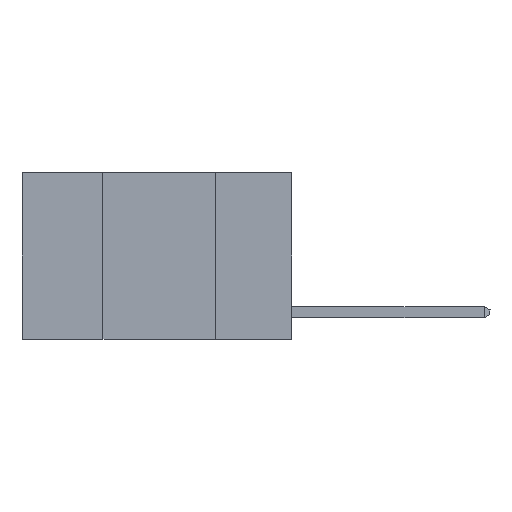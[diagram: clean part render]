
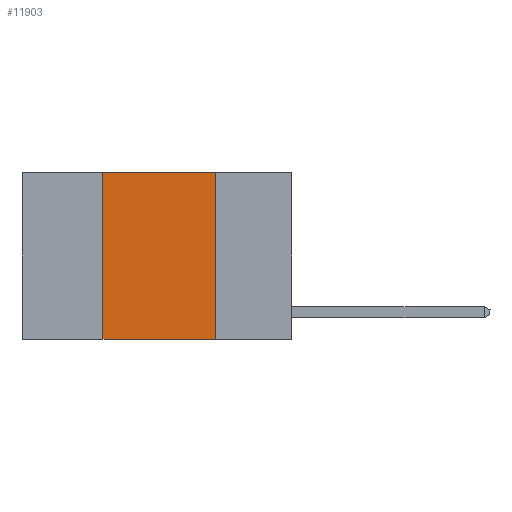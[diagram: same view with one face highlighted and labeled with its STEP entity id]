
A CAD part, left-side view. The second image highlights one B-rep face of the part: STEP entity #11903.
In plain terms, the highlighted planar face has unit normal (-1, 0, 0).
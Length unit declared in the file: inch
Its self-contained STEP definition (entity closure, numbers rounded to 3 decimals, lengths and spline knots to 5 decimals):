
#500 = LINE ( 'NONE', #10976, #11394 ) ;
#550 = ORIENTED_EDGE ( 'NONE', *, *, #27916, .F. ) ;
#1837 = CARTESIAN_POINT ( 'NONE',  ( 0., 0.6, 0. ) ) ;
#3663 = CARTESIAN_POINT ( 'NONE',  ( 0., 0.17, 0. ) ) ;
#4201 = VERTEX_POINT ( 'NONE', #20648 ) ;
#5074 = VECTOR ( 'NONE', #5381, 39.37008 ) ;
#5151 = PLANE ( 'NONE',  #21368 ) ;
#5301 = VERTEX_POINT ( 'NONE', #13723 ) ;
#5381 = DIRECTION ( 'NONE',  ( 0., 0., 1. ) ) ;
#5538 = EDGE_CURVE ( 'NONE', #4201, #11547, #6214, .T. ) ;
#6214 = LINE ( 'NONE', #3663, #17809 ) ;
#7266 = CARTESIAN_POINT ( 'NONE',  ( 0., 0.6, 0. ) ) ;
#9457 = DIRECTION ( 'NONE',  ( 1., 0., 0. ) ) ;
#10976 = CARTESIAN_POINT ( 'NONE',  ( 0., 0.6, -0.37 ) ) ;
#11394 = VECTOR ( 'NONE', #13148, 39.37008 ) ;
#11547 = VERTEX_POINT ( 'NONE', #16949 ) ;
#11903 = ADVANCED_FACE ( 'NONE', ( #14883 ), #5151, .F. ) ;
#12118 = ORIENTED_EDGE ( 'NONE', *, *, #5538, .F. ) ;
#12910 = EDGE_CURVE ( 'NONE', #5301, #11547, #500, .T. ) ;
#13148 = DIRECTION ( 'NONE',  ( 0., -1., 0. ) ) ;
#13723 = CARTESIAN_POINT ( 'NONE',  ( 0., 0.42, -0.37 ) ) ;
#14883 = FACE_OUTER_BOUND ( 'NONE', #27751, .T. ) ;
#14895 = DIRECTION ( 'NONE',  ( 0., -1., 0. ) ) ;
#16617 = LINE ( 'NONE', #20563, #5074 ) ;
#16949 = CARTESIAN_POINT ( 'NONE',  ( 0., 0.17, -0.37 ) ) ;
#17809 = VECTOR ( 'NONE', #18895, 39.37008 ) ;
#18363 = EDGE_CURVE ( 'NONE', #5301, #24720, #16617, .T. ) ;
#18895 = DIRECTION ( 'NONE',  ( 0., 0., -1. ) ) ;
#20198 = LINE ( 'NONE', #1837, #25943 ) ;
#20563 = CARTESIAN_POINT ( 'NONE',  ( 0., 0.42, 0. ) ) ;
#20648 = CARTESIAN_POINT ( 'NONE',  ( 0., 0.17, 0. ) ) ;
#21368 = AXIS2_PLACEMENT_3D ( 'NONE', #7266, #9457, #24659 ) ;
#24659 = DIRECTION ( 'NONE',  ( 0., 0., -1. ) ) ;
#24720 = VERTEX_POINT ( 'NONE', #25673 ) ;
#25070 = ORIENTED_EDGE ( 'NONE', *, *, #12910, .T. ) ;
#25673 = CARTESIAN_POINT ( 'NONE',  ( 0., 0.42, 0. ) ) ;
#25744 = ORIENTED_EDGE ( 'NONE', *, *, #18363, .F. ) ;
#25943 = VECTOR ( 'NONE', #14895, 39.37008 ) ;
#27751 = EDGE_LOOP ( 'NONE', ( #12118, #550, #25744, #25070 ) ) ;
#27916 = EDGE_CURVE ( 'NONE', #24720, #4201, #20198, .T. ) ;
